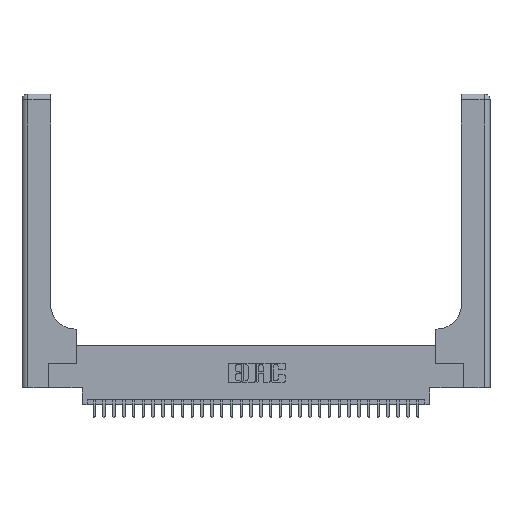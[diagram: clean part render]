
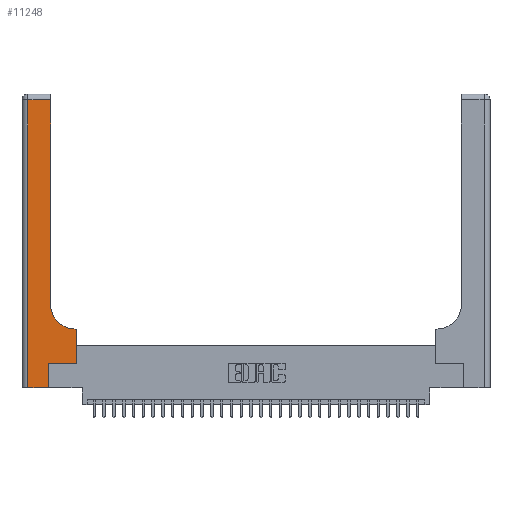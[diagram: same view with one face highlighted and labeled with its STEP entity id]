
A CAD part, top view. The second image highlights one B-rep face of the part: STEP entity #11248.
In plain terms, the highlighted planar face has unit normal (0, 0, 1).
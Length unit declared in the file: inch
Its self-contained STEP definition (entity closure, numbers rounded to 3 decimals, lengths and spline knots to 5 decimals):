
#606 = DIRECTION ( 'NONE',  ( 0., 0., -1. ) ) ;
#852 = EDGE_CURVE ( 'NONE', #26649, #18762, #5220, .T. ) ;
#2672 = EDGE_CURVE ( 'NONE', #29224, #9395, #14064, .T. ) ;
#2911 = DIRECTION ( 'NONE',  ( -1., 0., 0. ) ) ;
#3157 = CARTESIAN_POINT ( 'NONE',  ( 0.269, 0.25, 0.37 ) ) ;
#4333 = CARTESIAN_POINT ( 'NONE',  ( 0.2915, 0.6, 0.37 ) ) ;
#4500 = AXIS2_PLACEMENT_3D ( 'NONE', #26657, #606, #15792 ) ;
#4599 = CARTESIAN_POINT ( 'NONE',  ( 0.5415, 0.85, 0.37 ) ) ;
#4701 = ORIENTED_EDGE ( 'NONE', *, *, #21421, .T. ) ;
#5220 = LINE ( 'NONE', #13816, #8818 ) ;
#6004 = CARTESIAN_POINT ( 'NONE',  ( 0., 2.94, 0.37 ) ) ;
#6518 = CARTESIAN_POINT ( 'NONE',  ( 0.06, 2.94, 0.37 ) ) ;
#7457 = ORIENTED_EDGE ( 'NONE', *, *, #16735, .T. ) ;
#7499 = ORIENTED_EDGE ( 'NONE', *, *, #16224, .T. ) ;
#7558 = CARTESIAN_POINT ( 'NONE',  ( 0.06, 0., 0.37 ) ) ;
#7573 = LINE ( 'NONE', #22086, #27147 ) ;
#7927 = EDGE_LOOP ( 'NONE', ( #15413, #20786, #23406, #20967, #7457, #7499, #4701, #23325, #14854 ) ) ;
#7981 = CARTESIAN_POINT ( 'NONE',  ( 0.5585, 0.6, 0.37 ) ) ;
#8165 = LINE ( 'NONE', #29902, #19756 ) ;
#8315 = EDGE_CURVE ( 'NONE', #23987, #20346, #7573, .T. ) ;
#8728 = VERTEX_POINT ( 'NONE', #6518 ) ;
#8818 = VECTOR ( 'NONE', #28980, 39.37008 ) ;
#9395 = VERTEX_POINT ( 'NONE', #18745 ) ;
#9566 = CARTESIAN_POINT ( 'NONE',  ( 0.269, 0.25, 0.37 ) ) ;
#10109 = CARTESIAN_POINT ( 'NONE',  ( 0.2915, 2.94, 0.37 ) ) ;
#10114 = VECTOR ( 'NONE', #18963, 39.37008 ) ;
#10361 = PLANE ( 'NONE',  #4500 ) ;
#10818 = VECTOR ( 'NONE', #19683, 39.37008 ) ;
#11191 = AXIS2_PLACEMENT_3D ( 'NONE', #4599, #30408, #22238 ) ;
#11228 = CARTESIAN_POINT ( 'NONE',  ( 0.269, 0., 0.37 ) ) ;
#11248 = ADVANCED_FACE ( 'NONE', ( #30412 ), #10361, .F. ) ;
#11832 = LINE ( 'NONE', #6004, #15440 ) ;
#12478 = VERTEX_POINT ( 'NONE', #16985 ) ;
#13213 = CIRCLE ( 'NONE', #11191, 0.25 ) ;
#13816 = CARTESIAN_POINT ( 'NONE',  ( 0.2915, 3., 0.37 ) ) ;
#14064 = LINE ( 'NONE', #4333, #14892 ) ;
#14854 = ORIENTED_EDGE ( 'NONE', *, *, #18421, .T. ) ;
#14892 = VECTOR ( 'NONE', #2911, 39.37008 ) ;
#15413 = ORIENTED_EDGE ( 'NONE', *, *, #852, .T. ) ;
#15416 = VECTOR ( 'NONE', #21049, 39.37008 ) ;
#15440 = VECTOR ( 'NONE', #26445, 39.37008 ) ;
#15792 = DIRECTION ( 'NONE',  ( -1., 0., 0. ) ) ;
#16224 = EDGE_CURVE ( 'NONE', #30746, #12478, #23732, .T. ) ;
#16735 = EDGE_CURVE ( 'NONE', #20346, #30746, #19328, .T. ) ;
#16985 = CARTESIAN_POINT ( 'NONE',  ( 0.5585, 0.25, 0.37 ) ) ;
#18421 = EDGE_CURVE ( 'NONE', #9395, #26649, #13213, .T. ) ;
#18745 = CARTESIAN_POINT ( 'NONE',  ( 0.5415, 0.6, 0.37 ) ) ;
#18762 = VERTEX_POINT ( 'NONE', #10109 ) ;
#18866 = LINE ( 'NONE', #22679, #10818 ) ;
#18963 = DIRECTION ( 'NONE',  ( 0., 1., 0. ) ) ;
#19183 = DIRECTION ( 'NONE',  ( 1., 0., 0. ) ) ;
#19328 = LINE ( 'NONE', #11228, #10114 ) ;
#19683 = DIRECTION ( 'NONE',  ( 0., -1., 0. ) ) ;
#19756 = VECTOR ( 'NONE', #32105, 39.37008 ) ;
#20346 = VERTEX_POINT ( 'NONE', #22344 ) ;
#20786 = ORIENTED_EDGE ( 'NONE', *, *, #32920, .T. ) ;
#20967 = ORIENTED_EDGE ( 'NONE', *, *, #8315, .T. ) ;
#21049 = DIRECTION ( 'NONE',  ( 1., 0., 0. ) ) ;
#21421 = EDGE_CURVE ( 'NONE', #12478, #29224, #8165, .T. ) ;
#22086 = CARTESIAN_POINT ( 'NONE',  ( 0., 0., 0.37 ) ) ;
#22238 = DIRECTION ( 'NONE',  ( 1., 0., 0. ) ) ;
#22344 = CARTESIAN_POINT ( 'NONE',  ( 0.269, 0., 0.37 ) ) ;
#22419 = CARTESIAN_POINT ( 'NONE',  ( 0.2915, 0.85, 0.37 ) ) ;
#22679 = CARTESIAN_POINT ( 'NONE',  ( 0.06, 3., 0.37 ) ) ;
#23325 = ORIENTED_EDGE ( 'NONE', *, *, #2672, .T. ) ;
#23406 = ORIENTED_EDGE ( 'NONE', *, *, #24180, .T. ) ;
#23732 = LINE ( 'NONE', #3157, #15416 ) ;
#23987 = VERTEX_POINT ( 'NONE', #7558 ) ;
#24180 = EDGE_CURVE ( 'NONE', #8728, #23987, #18866, .T. ) ;
#26445 = DIRECTION ( 'NONE',  ( -1., 0., 0. ) ) ;
#26649 = VERTEX_POINT ( 'NONE', #22419 ) ;
#26657 = CARTESIAN_POINT ( 'NONE',  ( 0., 3., 0.37 ) ) ;
#27147 = VECTOR ( 'NONE', #19183, 39.37008 ) ;
#28980 = DIRECTION ( 'NONE',  ( 0., 1., 0. ) ) ;
#29224 = VERTEX_POINT ( 'NONE', #7981 ) ;
#29902 = CARTESIAN_POINT ( 'NONE',  ( 0.5585, 0.25, 0.37 ) ) ;
#30408 = DIRECTION ( 'NONE',  ( 0., 0., -1. ) ) ;
#30412 = FACE_OUTER_BOUND ( 'NONE', #7927, .T. ) ;
#30746 = VERTEX_POINT ( 'NONE', #9566 ) ;
#32105 = DIRECTION ( 'NONE',  ( 0., 1., 0. ) ) ;
#32920 = EDGE_CURVE ( 'NONE', #18762, #8728, #11832, .T. ) ;
